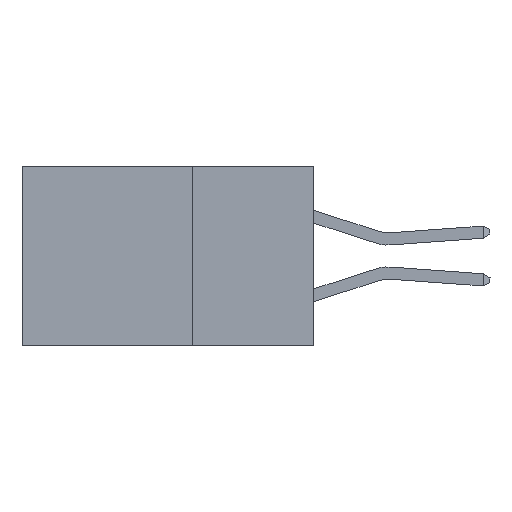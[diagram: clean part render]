
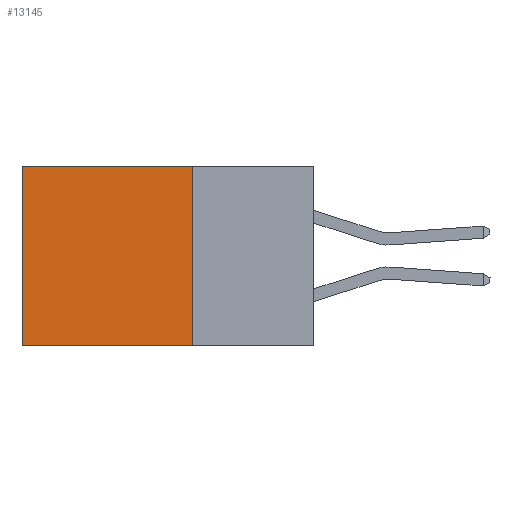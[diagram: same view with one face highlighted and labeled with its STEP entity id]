
A CAD part, left-side view. The second image highlights one B-rep face of the part: STEP entity #13145.
In plain terms, the highlighted planar face has unit normal (-1, 0, 0).
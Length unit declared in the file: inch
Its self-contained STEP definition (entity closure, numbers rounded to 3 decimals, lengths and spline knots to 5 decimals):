
#295 = LINE ( 'NONE', #13545, #42073 ) ;
#657 = LINE ( 'NONE', #19623, #33723 ) ;
#2113 = ORIENTED_EDGE ( 'NONE', *, *, #18079, .F. ) ;
#3254 = CARTESIAN_POINT ( 'NONE',  ( 0.2875, 0.25, -0.37 ) ) ;
#6897 = DIRECTION ( 'NONE',  ( 0., 1., 0. ) ) ;
#8518 = EDGE_CURVE ( 'NONE', #17775, #31998, #657, .T. ) ;
#11255 = EDGE_CURVE ( 'NONE', #26604, #19326, #36051, .T. ) ;
#12216 = ORIENTED_EDGE ( 'NONE', *, *, #11255, .F. ) ;
#13145 = ADVANCED_FACE ( 'NONE', ( #21469 ), #32509, .F. ) ;
#13545 = CARTESIAN_POINT ( 'NONE',  ( 0.2875, 0.25, 0. ) ) ;
#16254 = DIRECTION ( 'NONE',  ( 0., 0., -1. ) ) ;
#17028 = EDGE_LOOP ( 'NONE', ( #21257, #2113, #12216, #31603 ) ) ;
#17775 = VERTEX_POINT ( 'NONE', #18156 ) ;
#18079 = EDGE_CURVE ( 'NONE', #19326, #31998, #21922, .T. ) ;
#18156 = CARTESIAN_POINT ( 'NONE',  ( 0.2875, 0.6, 0. ) ) ;
#19326 = VERTEX_POINT ( 'NONE', #22391 ) ;
#19623 = CARTESIAN_POINT ( 'NONE',  ( 0.2875, 0.6, 0. ) ) ;
#19770 = AXIS2_PLACEMENT_3D ( 'NONE', #29215, #42256, #35822 ) ;
#21257 = ORIENTED_EDGE ( 'NONE', *, *, #8518, .T. ) ;
#21469 = FACE_OUTER_BOUND ( 'NONE', #17028, .T. ) ;
#21828 = EDGE_CURVE ( 'NONE', #26604, #17775, #295, .T. ) ;
#21922 = LINE ( 'NONE', #3254, #40428 ) ;
#22391 = CARTESIAN_POINT ( 'NONE',  ( 0.2875, 0.25, -0.37 ) ) ;
#26355 = DIRECTION ( 'NONE',  ( 0., 1., 0. ) ) ;
#26604 = VERTEX_POINT ( 'NONE', #31066 ) ;
#27347 = VECTOR ( 'NONE', #16254, 39.37008 ) ;
#29215 = CARTESIAN_POINT ( 'NONE',  ( 0.2875, 0.25, 0. ) ) ;
#31066 = CARTESIAN_POINT ( 'NONE',  ( 0.2875, 0.25, 0. ) ) ;
#31603 = ORIENTED_EDGE ( 'NONE', *, *, #21828, .T. ) ;
#31998 = VERTEX_POINT ( 'NONE', #41987 ) ;
#32509 = PLANE ( 'NONE',  #19770 ) ;
#33723 = VECTOR ( 'NONE', #42598, 39.37008 ) ;
#35822 = DIRECTION ( 'NONE',  ( 0., 0., -1. ) ) ;
#35956 = CARTESIAN_POINT ( 'NONE',  ( 0.2875, 0.25, 0. ) ) ;
#36051 = LINE ( 'NONE', #35956, #27347 ) ;
#40428 = VECTOR ( 'NONE', #26355, 39.37008 ) ;
#41987 = CARTESIAN_POINT ( 'NONE',  ( 0.2875, 0.6, -0.37 ) ) ;
#42073 = VECTOR ( 'NONE', #6897, 39.37008 ) ;
#42256 = DIRECTION ( 'NONE',  ( 1., 0., 0. ) ) ;
#42598 = DIRECTION ( 'NONE',  ( 0., 0., -1. ) ) ;
